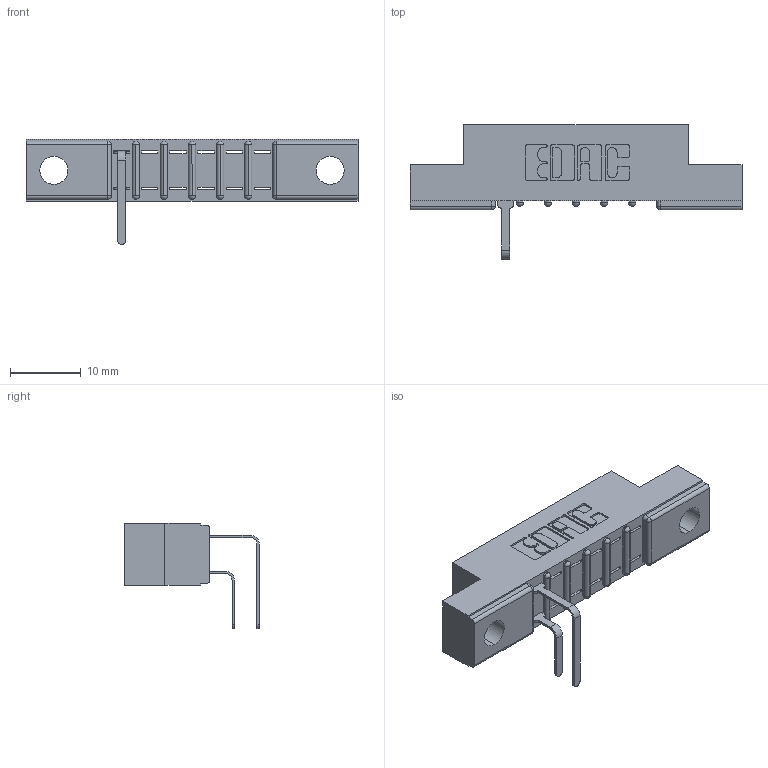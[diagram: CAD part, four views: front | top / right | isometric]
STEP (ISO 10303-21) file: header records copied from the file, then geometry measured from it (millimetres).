
FILE_DESCRIPTION (( 'STEP AP203' ), '1' );
FILE_NAME ('357-006-558-104.STEP', '2018-08-06T22:57:05', ( '' ), ( '' ), 'SwSTEP 2.0', 'SolidWorks 2016', '' );
FILE_SCHEMA (( 'CONFIG_CONTROL_DESIGN' ));
Length unit declared in the file: inch
Products named in the file (4): 357-006-558-104; 307 Part_.156 Dia Mounting Holes; 307-290-001_558 559 - 1 (Single); 307-290-001_558 - 2 (Single)
Assembly tree (3 placements, depth 2):
  357-006-558-104
    307 Part_.156 Dia Mounting Holes
    307-290-001_558 559 - 1 (Single)
    307-290-001_558 - 2 (Single)
Bounding box: 46.79 x 18.96 x 14.81 mm (x, y, z)
Volume: 2835.6 mm3; surface area: 3347.8 mm2
Topology: 3 solids, 3 shells, 339 faces, 963 edges, 618 vertices
Faces by surface type: plane 210, cylinder 115, sphere 14
Entity records: 11319 total; most frequent: CARTESIAN_POINT 1912, ORIENTED_EDGE 1898, DIRECTION 1869, EDGE_CURVE 949, VECTOR 719, LINE 719, VERTEX_POINT 618, AXIS2_PLACEMENT_3D 575
